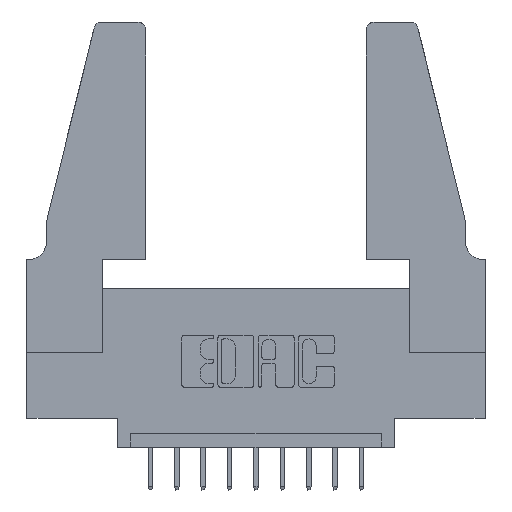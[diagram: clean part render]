
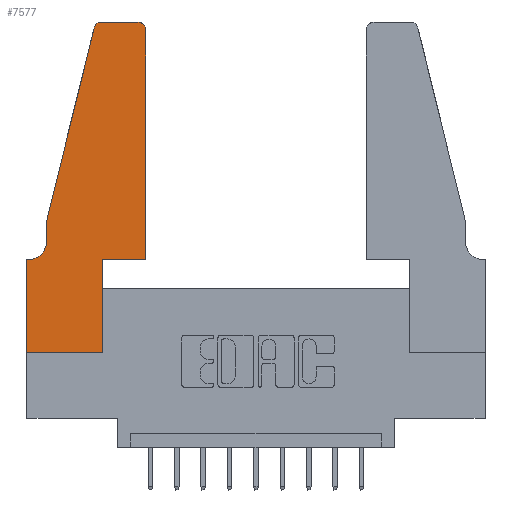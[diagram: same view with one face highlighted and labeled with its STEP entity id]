
A CAD part, top view. The second image highlights one B-rep face of the part: STEP entity #7577.
In plain terms, the highlighted planar face has unit normal (0, 0, 1).
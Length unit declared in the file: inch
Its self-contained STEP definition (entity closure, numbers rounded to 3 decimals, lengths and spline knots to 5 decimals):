
#4 = DIRECTION ( 'NONE',  ( 0., 1., 0. ) ) ;
#460 = CIRCLE ( 'NONE', #8711, 0.03 ) ;
#582 = ORIENTED_EDGE ( 'NONE', *, *, #13420, .T. ) ;
#769 = DIRECTION ( 'NONE',  ( 0., 0., 1. ) ) ;
#848 = CARTESIAN_POINT ( 'NONE',  ( 0., 0.35, 0.37 ) ) ;
#859 = EDGE_CURVE ( 'NONE', #5911, #11658, #12597, .T. ) ;
#968 = EDGE_CURVE ( 'NONE', #8944, #1265, #460, .T. ) ;
#1087 = EDGE_CURVE ( 'NONE', #5250, #7210, #7887, .T. ) ;
#1140 = DIRECTION ( 'NONE',  ( -1., 0., 0. ) ) ;
#1265 = VERTEX_POINT ( 'NONE', #13546 ) ;
#1281 = DIRECTION ( 'NONE',  ( 0., 0., 1. ) ) ;
#1326 = ORIENTED_EDGE ( 'NONE', *, *, #1087, .T. ) ;
#1350 = AXIS2_PLACEMENT_3D ( 'NONE', #848, #769, #8247 ) ;
#1385 = LINE ( 'NONE', #4956, #5674 ) ;
#1401 = EDGE_CURVE ( 'NONE', #7210, #4054, #4367, .T. ) ;
#1548 = CARTESIAN_POINT ( 'NONE',  ( 0., 0., 0.37 ) ) ;
#1760 = EDGE_CURVE ( 'NONE', #2283, #5911, #10454, .T. ) ;
#2283 = VERTEX_POINT ( 'NONE', #12669 ) ;
#2508 = CARTESIAN_POINT ( 'NONE',  ( 0.4205, 1.22, 0.37 ) ) ;
#2622 = LINE ( 'NONE', #3147, #9524 ) ;
#2774 = EDGE_CURVE ( 'NONE', #11658, #3337, #1385, .T. ) ;
#2895 = AXIS2_PLACEMENT_3D ( 'NONE', #3204, #4172, #1140 ) ;
#2958 = CARTESIAN_POINT ( 'NONE',  ( 0., 0.35, 0.37 ) ) ;
#3147 = CARTESIAN_POINT ( 'NONE',  ( 0.0755, 0.5, 0.37 ) ) ;
#3204 = CARTESIAN_POINT ( 'NONE',  ( 0.0055, 0.42, 0.37 ) ) ;
#3337 = VERTEX_POINT ( 'NONE', #2958 ) ;
#3345 = ORIENTED_EDGE ( 'NONE', *, *, #2774, .T. ) ;
#3381 = CARTESIAN_POINT ( 'NONE',  ( 0.284, 1.25, 0.37 ) ) ;
#4054 = VERTEX_POINT ( 'NONE', #4148 ) ;
#4148 = CARTESIAN_POINT ( 'NONE',  ( 0.4505, 0.35, 0.37 ) ) ;
#4172 = DIRECTION ( 'NONE',  ( 0., 0., -1. ) ) ;
#4367 = LINE ( 'NONE', #10645, #7356 ) ;
#4717 = ORIENTED_EDGE ( 'NONE', *, *, #13296, .T. ) ;
#4860 = DIRECTION ( 'NONE',  ( 1., 0., 0. ) ) ;
#4956 = CARTESIAN_POINT ( 'NONE',  ( 0.0755, 0.35, 0.37 ) ) ;
#5250 = VERTEX_POINT ( 'NONE', #5310 ) ;
#5310 = CARTESIAN_POINT ( 'NONE',  ( 0.2865, 0., 0.37 ) ) ;
#5314 = CARTESIAN_POINT ( 'NONE',  ( 0.4505, 0.35, 0.37 ) ) ;
#5600 = EDGE_CURVE ( 'NONE', #4054, #8944, #10933, .T. ) ;
#5674 = VECTOR ( 'NONE', #8171, 39.37008 ) ;
#5911 = VERTEX_POINT ( 'NONE', #11454 ) ;
#6023 = VERTEX_POINT ( 'NONE', #3381 ) ;
#6035 = PLANE ( 'NONE',  #1350 ) ;
#6084 = DIRECTION ( 'NONE',  ( 0., 0., 1. ) ) ;
#6094 = ORIENTED_EDGE ( 'NONE', *, *, #11617, .T. ) ;
#6123 = ORIENTED_EDGE ( 'NONE', *, *, #5600, .T. ) ;
#6496 = ORIENTED_EDGE ( 'NONE', *, *, #968, .T. ) ;
#6513 = VERTEX_POINT ( 'NONE', #13342 ) ;
#6919 = DIRECTION ( 'NONE',  ( 0., 1., 0. ) ) ;
#7210 = VERTEX_POINT ( 'NONE', #7704 ) ;
#7341 = DIRECTION ( 'NONE',  ( 0., -1., 0. ) ) ;
#7356 = VECTOR ( 'NONE', #11696, 39.37008 ) ;
#7532 = VECTOR ( 'NONE', #7960, 39.37008 ) ;
#7577 = ADVANCED_FACE ( 'NONE', ( #9567 ), #6035, .T. ) ;
#7646 = CARTESIAN_POINT ( 'NONE',  ( 0.2605, 1.25, 0.37 ) ) ;
#7678 = VECTOR ( 'NONE', #7341, 39.37008 ) ;
#7704 = CARTESIAN_POINT ( 'NONE',  ( 0.2865, 0.35, 0.37 ) ) ;
#7887 = LINE ( 'NONE', #10985, #10810 ) ;
#7960 = DIRECTION ( 'NONE',  ( 0., -1., 0. ) ) ;
#8171 = DIRECTION ( 'NONE',  ( -1., 0., 0. ) ) ;
#8217 = EDGE_CURVE ( 'NONE', #6513, #5250, #8402, .T. ) ;
#8239 = CARTESIAN_POINT ( 'NONE',  ( 0.0755, 0.5, 0.37 ) ) ;
#8247 = DIRECTION ( 'NONE',  ( 1., 0., 0. ) ) ;
#8402 = LINE ( 'NONE', #8955, #12785 ) ;
#8711 = AXIS2_PLACEMENT_3D ( 'NONE', #2508, #1281, #12745 ) ;
#8944 = VERTEX_POINT ( 'NONE', #10870 ) ;
#8955 = CARTESIAN_POINT ( 'NONE',  ( 0., 0., 0.37 ) ) ;
#9008 = ORIENTED_EDGE ( 'NONE', *, *, #8217, .T. ) ;
#9524 = VECTOR ( 'NONE', #10462, 39.37008 ) ;
#9542 = EDGE_CURVE ( 'NONE', #1265, #6023, #11455, .T. ) ;
#9567 = FACE_OUTER_BOUND ( 'NONE', #11378, .T. ) ;
#9909 = CARTESIAN_POINT ( 'NONE',  ( 0.25487, 1.22718, 0.37 ) ) ;
#10018 = LINE ( 'NONE', #1548, #7532 ) ;
#10436 = ORIENTED_EDGE ( 'NONE', *, *, #1760, .T. ) ;
#10454 = LINE ( 'NONE', #8239, #7678 ) ;
#10462 = DIRECTION ( 'NONE',  ( -0.239, -0.971, 0. ) ) ;
#10569 = VECTOR ( 'NONE', #4, 39.37008 ) ;
#10645 = CARTESIAN_POINT ( 'NONE',  ( 0.4505, 0.35, 0.37 ) ) ;
#10810 = VECTOR ( 'NONE', #6919, 39.37008 ) ;
#10870 = CARTESIAN_POINT ( 'NONE',  ( 0.4505, 1.22, 0.37 ) ) ;
#10933 = LINE ( 'NONE', #5314, #10569 ) ;
#10985 = CARTESIAN_POINT ( 'NONE',  ( 0.2865, 0.35, 0.37 ) ) ;
#11092 = CARTESIAN_POINT ( 'NONE',  ( 0.0055, 0.35, 0.37 ) ) ;
#11378 = EDGE_LOOP ( 'NONE', ( #11913, #6094, #582, #10436, #12507, #3345, #4717, #9008, #1326, #12788, #6123, #6496 ) ) ;
#11454 = CARTESIAN_POINT ( 'NONE',  ( 0.0755, 0.42, 0.37 ) ) ;
#11455 = LINE ( 'NONE', #7646, #13547 ) ;
#11617 = EDGE_CURVE ( 'NONE', #6023, #12181, #13288, .T. ) ;
#11658 = VERTEX_POINT ( 'NONE', #11092 ) ;
#11676 = DIRECTION ( 'NONE',  ( -1., 0., 0. ) ) ;
#11696 = DIRECTION ( 'NONE',  ( 1., 0., 0. ) ) ;
#11913 = ORIENTED_EDGE ( 'NONE', *, *, #9542, .T. ) ;
#12181 = VERTEX_POINT ( 'NONE', #9909 ) ;
#12507 = ORIENTED_EDGE ( 'NONE', *, *, #859, .T. ) ;
#12597 = CIRCLE ( 'NONE', #2895, 0.07 ) ;
#12669 = CARTESIAN_POINT ( 'NONE',  ( 0.0755, 0.5, 0.37 ) ) ;
#12745 = DIRECTION ( 'NONE',  ( 1., 0., 0. ) ) ;
#12785 = VECTOR ( 'NONE', #4860, 39.37008 ) ;
#12788 = ORIENTED_EDGE ( 'NONE', *, *, #1401, .T. ) ;
#12897 = AXIS2_PLACEMENT_3D ( 'NONE', #13167, #6084, #13379 ) ;
#13167 = CARTESIAN_POINT ( 'NONE',  ( 0.284, 1.22, 0.37 ) ) ;
#13288 = CIRCLE ( 'NONE', #12897, 0.03 ) ;
#13296 = EDGE_CURVE ( 'NONE', #3337, #6513, #10018, .T. ) ;
#13342 = CARTESIAN_POINT ( 'NONE',  ( 0., 0., 0.37 ) ) ;
#13379 = DIRECTION ( 'NONE',  ( 1., 0., 0. ) ) ;
#13420 = EDGE_CURVE ( 'NONE', #12181, #2283, #2622, .T. ) ;
#13546 = CARTESIAN_POINT ( 'NONE',  ( 0.4205, 1.25, 0.37 ) ) ;
#13547 = VECTOR ( 'NONE', #11676, 39.37008 ) ;
